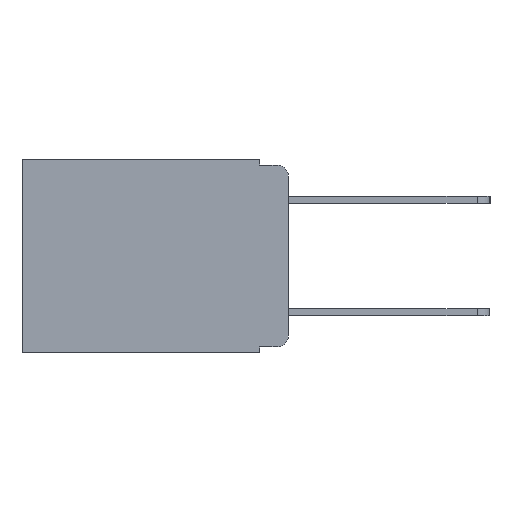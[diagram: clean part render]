
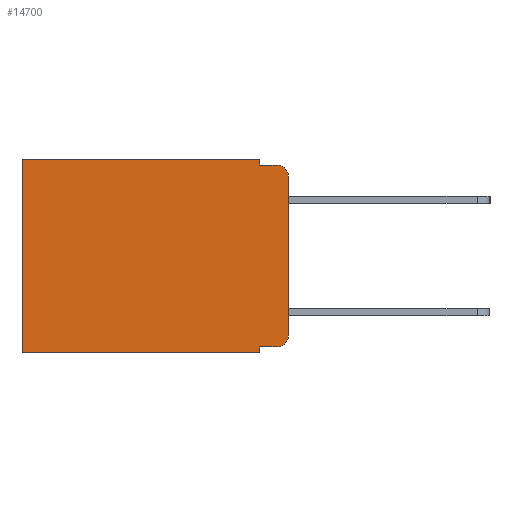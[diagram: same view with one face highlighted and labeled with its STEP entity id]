
A CAD part, left-side view. The second image highlights one B-rep face of the part: STEP entity #14700.
In plain terms, the highlighted planar face has unit normal (-1, 0, 0).
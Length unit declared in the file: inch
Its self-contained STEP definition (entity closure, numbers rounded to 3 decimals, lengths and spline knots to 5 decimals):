
#27 = VECTOR ( 'NONE', #1866, 39.37008 ) ;
#209 = VECTOR ( 'NONE', #6300, 39.37008 ) ;
#295 = LINE ( 'NONE', #14433, #8061 ) ;
#609 = EDGE_CURVE ( 'NONE', #6720, #9598, #18188, .T. ) ;
#672 = VECTOR ( 'NONE', #3661, 39.37008 ) ;
#1040 = ORIENTED_EDGE ( 'NONE', *, *, #12133, .T. ) ;
#1317 = VERTEX_POINT ( 'NONE', #16462 ) ;
#1603 = CARTESIAN_POINT ( 'NONE',  ( 0.298, 0.473, 0. ) ) ;
#1866 = DIRECTION ( 'NONE',  ( 0., -1., 0. ) ) ;
#2020 = ORIENTED_EDGE ( 'NONE', *, *, #11284, .F. ) ;
#2239 = EDGE_CURVE ( 'NONE', #1317, #8706, #12486, .T. ) ;
#2339 = CARTESIAN_POINT ( 'NONE',  ( 0.298, 0., -0.313 ) ) ;
#2515 = VECTOR ( 'NONE', #15780, 39.37008 ) ;
#2890 = VERTEX_POINT ( 'NONE', #10729 ) ;
#3012 = FACE_OUTER_BOUND ( 'NONE', #6668, .T. ) ;
#3033 = DIRECTION ( 'NONE',  ( 0., 0., -1. ) ) ;
#3406 = DIRECTION ( 'NONE',  ( -1., 0., 0. ) ) ;
#3471 = VECTOR ( 'NONE', #11433, 39.37008 ) ;
#3661 = DIRECTION ( 'NONE',  ( 0., -1., 0. ) ) ;
#3792 = EDGE_CURVE ( 'NONE', #15502, #15758, #14652, .T. ) ;
#4659 = AXIS2_PLACEMENT_3D ( 'NONE', #16143, #8237, #17404 ) ;
#5055 = CARTESIAN_POINT ( 'NONE',  ( 0.298, 0.051, -0.343 ) ) ;
#5271 = VERTEX_POINT ( 'NONE', #5946 ) ;
#5452 = CARTESIAN_POINT ( 'NONE',  ( 0.298, 0., 0. ) ) ;
#5812 = CARTESIAN_POINT ( 'NONE',  ( 0.298, 0.473, -0.343 ) ) ;
#5946 = CARTESIAN_POINT ( 'NONE',  ( 0.298, 0.473, 0. ) ) ;
#6143 = CARTESIAN_POINT ( 'NONE',  ( 0.298, 0.051, -0.01 ) ) ;
#6212 = ORIENTED_EDGE ( 'NONE', *, *, #2239, .F. ) ;
#6253 = DIRECTION ( 'NONE',  ( 0., 1., 0. ) ) ;
#6300 = DIRECTION ( 'NONE',  ( 0., 0., -1. ) ) ;
#6668 = EDGE_LOOP ( 'NONE', ( #14135, #1040, #14974, #6212, #11488, #17115, #8714, #2020, #12543, #14759 ) ) ;
#6720 = VERTEX_POINT ( 'NONE', #14574 ) ;
#6795 = EDGE_CURVE ( 'NONE', #8706, #2890, #8309, .T. ) ;
#6961 = DIRECTION ( 'NONE',  ( 0., 0., -1. ) ) ;
#7427 = VERTEX_POINT ( 'NONE', #5055 ) ;
#8061 = VECTOR ( 'NONE', #6253, 39.37008 ) ;
#8176 = CIRCLE ( 'NONE', #9613, 0.02 ) ;
#8237 = DIRECTION ( 'NONE',  ( -1., 0., 0. ) ) ;
#8309 = LINE ( 'NONE', #12117, #27 ) ;
#8533 = VERTEX_POINT ( 'NONE', #5812 ) ;
#8706 = VERTEX_POINT ( 'NONE', #6143 ) ;
#8714 = ORIENTED_EDGE ( 'NONE', *, *, #9294, .F. ) ;
#8817 = CARTESIAN_POINT ( 'NONE',  ( 0.298, 0.051, -0.333 ) ) ;
#9294 = EDGE_CURVE ( 'NONE', #7427, #8533, #295, .T. ) ;
#9430 = DIRECTION ( 'NONE',  ( 0., 0., -1. ) ) ;
#9598 = VERTEX_POINT ( 'NONE', #2339 ) ;
#9613 = AXIS2_PLACEMENT_3D ( 'NONE', #12037, #3406, #13367 ) ;
#9729 = CIRCLE ( 'NONE', #4659, 0.02 ) ;
#10709 = EDGE_CURVE ( 'NONE', #5271, #8533, #16888, .T. ) ;
#10729 = CARTESIAN_POINT ( 'NONE',  ( 0.298, 0.02, -0.01 ) ) ;
#10963 = CARTESIAN_POINT ( 'NONE',  ( 0.298, 0.051, -0.333 ) ) ;
#11104 = PLANE ( 'NONE',  #11768 ) ;
#11207 = LINE ( 'NONE', #16607, #3471 ) ;
#11284 = EDGE_CURVE ( 'NONE', #15502, #7427, #18228, .T. ) ;
#11433 = DIRECTION ( 'NONE',  ( 0., 1., 0. ) ) ;
#11488 = ORIENTED_EDGE ( 'NONE', *, *, #15485, .T. ) ;
#11768 = AXIS2_PLACEMENT_3D ( 'NONE', #5452, #15046, #6961 ) ;
#12037 = CARTESIAN_POINT ( 'NONE',  ( 0.298, 0.02, -0.03 ) ) ;
#12117 = CARTESIAN_POINT ( 'NONE',  ( 0.298, 0.051, -0.01 ) ) ;
#12133 = EDGE_CURVE ( 'NONE', #6720, #2890, #8176, .T. ) ;
#12486 = LINE ( 'NONE', #16960, #209 ) ;
#12543 = ORIENTED_EDGE ( 'NONE', *, *, #3792, .T. ) ;
#13046 = CARTESIAN_POINT ( 'NONE',  ( 0.298, 0.051, 0. ) ) ;
#13367 = DIRECTION ( 'NONE',  ( 0., 0., -1. ) ) ;
#14135 = ORIENTED_EDGE ( 'NONE', *, *, #609, .F. ) ;
#14433 = CARTESIAN_POINT ( 'NONE',  ( 0.298, 0., -0.343 ) ) ;
#14574 = CARTESIAN_POINT ( 'NONE',  ( 0.298, 0., -0.03 ) ) ;
#14652 = LINE ( 'NONE', #10963, #672 ) ;
#14700 = ADVANCED_FACE ( 'NONE', ( #3012 ), #11104, .F. ) ;
#14731 = CARTESIAN_POINT ( 'NONE',  ( 0.298, 0.02, -0.333 ) ) ;
#14759 = ORIENTED_EDGE ( 'NONE', *, *, #17519, .T. ) ;
#14974 = ORIENTED_EDGE ( 'NONE', *, *, #6795, .F. ) ;
#15046 = DIRECTION ( 'NONE',  ( 1., 0., 0. ) ) ;
#15247 = VECTOR ( 'NONE', #9430, 39.37008 ) ;
#15283 = VECTOR ( 'NONE', #3033, 39.37008 ) ;
#15485 = EDGE_CURVE ( 'NONE', #1317, #5271, #11207, .T. ) ;
#15502 = VERTEX_POINT ( 'NONE', #8817 ) ;
#15758 = VERTEX_POINT ( 'NONE', #14731 ) ;
#15780 = DIRECTION ( 'NONE',  ( 0., 0., -1. ) ) ;
#16023 = CARTESIAN_POINT ( 'NONE',  ( 0.298, 0., 0. ) ) ;
#16143 = CARTESIAN_POINT ( 'NONE',  ( 0.298, 0.02, -0.313 ) ) ;
#16462 = CARTESIAN_POINT ( 'NONE',  ( 0.298, 0.051, 0. ) ) ;
#16607 = CARTESIAN_POINT ( 'NONE',  ( 0.298, 0., 0. ) ) ;
#16888 = LINE ( 'NONE', #1603, #2515 ) ;
#16960 = CARTESIAN_POINT ( 'NONE',  ( 0.298, 0.051, 0. ) ) ;
#17115 = ORIENTED_EDGE ( 'NONE', *, *, #10709, .T. ) ;
#17404 = DIRECTION ( 'NONE',  ( 0., 0., -1. ) ) ;
#17519 = EDGE_CURVE ( 'NONE', #15758, #9598, #9729, .T. ) ;
#18188 = LINE ( 'NONE', #16023, #15247 ) ;
#18228 = LINE ( 'NONE', #13046, #15283 ) ;
